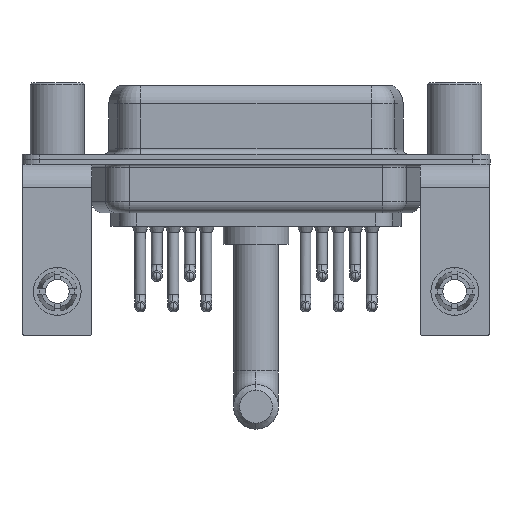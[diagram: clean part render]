
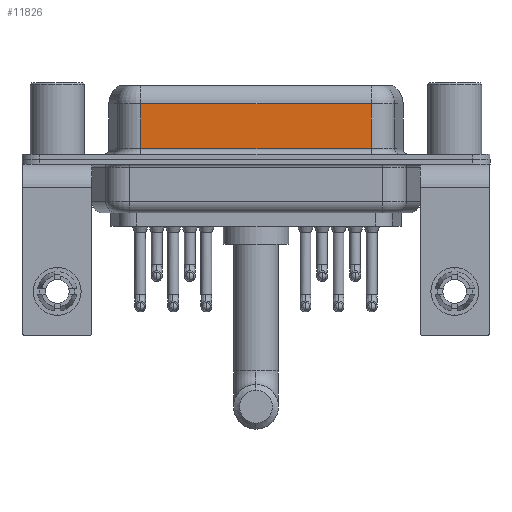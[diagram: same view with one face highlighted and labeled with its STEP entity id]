
A CAD part, front view. The second image highlights one B-rep face of the part: STEP entity #11826.
In plain terms, the highlighted planar face has unit normal (0, -1, 0).
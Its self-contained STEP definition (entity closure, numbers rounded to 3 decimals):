
#396 = CARTESIAN_POINT ( 'NONE',  ( 26.287, -3.95, 6.4 ) ) ;
#1691 = DIRECTION ( 'NONE',  ( 0., 1., 0. ) ) ;
#2332 = CARTESIAN_POINT ( 'NONE',  ( 26.287, -3.95, 0.9 ) ) ;
#2859 = VERTEX_POINT ( 'NONE', #22129 ) ;
#3455 = ORIENTED_EDGE ( 'NONE', *, *, #15270, .T. ) ;
#4665 = LINE ( 'NONE', #22220, #11291 ) ;
#4693 = LINE ( 'NONE', #11715, #20842 ) ;
#4807 = ORIENTED_EDGE ( 'NONE', *, *, #6831, .T. ) ;
#5285 = CARTESIAN_POINT ( 'NONE',  ( 26.287, -3.95, 6.4 ) ) ;
#6027 = ORIENTED_EDGE ( 'NONE', *, *, #8072, .T. ) ;
#6473 = AXIS2_PLACEMENT_3D ( 'NONE', #5285, #1691, #19151 ) ;
#6755 = DIRECTION ( 'NONE',  ( -1., 0., 0. ) ) ;
#6831 = EDGE_CURVE ( 'NONE', #2859, #9576, #11199, .T. ) ;
#7876 = CARTESIAN_POINT ( 'NONE',  ( 7.013, -3.95, 4.65 ) ) ;
#8072 = EDGE_CURVE ( 'NONE', #21669, #16668, #4693, .T. ) ;
#8158 = EDGE_CURVE ( 'NONE', #21669, #9576, #19569, .T. ) ;
#8781 = EDGE_LOOP ( 'NONE', ( #13883, #6027, #3455, #4807 ) ) ;
#9246 = CARTESIAN_POINT ( 'NONE',  ( 26.287, -3.95, 0.9 ) ) ;
#9576 = VERTEX_POINT ( 'NONE', #9246 ) ;
#11199 = LINE ( 'NONE', #2332, #18316 ) ;
#11291 = VECTOR ( 'NONE', #11686, 1000. ) ;
#11686 = DIRECTION ( 'NONE',  ( 0., 0., -1. ) ) ;
#11715 = CARTESIAN_POINT ( 'NONE',  ( 26.287, -3.95, 4.65 ) ) ;
#11826 = ADVANCED_FACE ( 'NONE', ( #14124 ), #19261, .F. ) ;
#13883 = ORIENTED_EDGE ( 'NONE', *, *, #8158, .F. ) ;
#14124 = FACE_OUTER_BOUND ( 'NONE', #8781, .T. ) ;
#15270 = EDGE_CURVE ( 'NONE', #16668, #2859, #4665, .T. ) ;
#16668 = VERTEX_POINT ( 'NONE', #7876 ) ;
#16686 = VECTOR ( 'NONE', #19337, 1000. ) ;
#17909 = DIRECTION ( 'NONE',  ( 1., 0., 0. ) ) ;
#18316 = VECTOR ( 'NONE', #17909, 1000. ) ;
#18486 = CARTESIAN_POINT ( 'NONE',  ( 26.287, -3.95, 4.65 ) ) ;
#19151 = DIRECTION ( 'NONE',  ( 0., 0., 1. ) ) ;
#19261 = PLANE ( 'NONE',  #6473 ) ;
#19337 = DIRECTION ( 'NONE',  ( 0., 0., -1. ) ) ;
#19569 = LINE ( 'NONE', #396, #16686 ) ;
#20842 = VECTOR ( 'NONE', #6755, 1000. ) ;
#21669 = VERTEX_POINT ( 'NONE', #18486 ) ;
#22129 = CARTESIAN_POINT ( 'NONE',  ( 7.013, -3.95, 0.9 ) ) ;
#22220 = CARTESIAN_POINT ( 'NONE',  ( 7.013, -3.95, 6.4 ) ) ;
